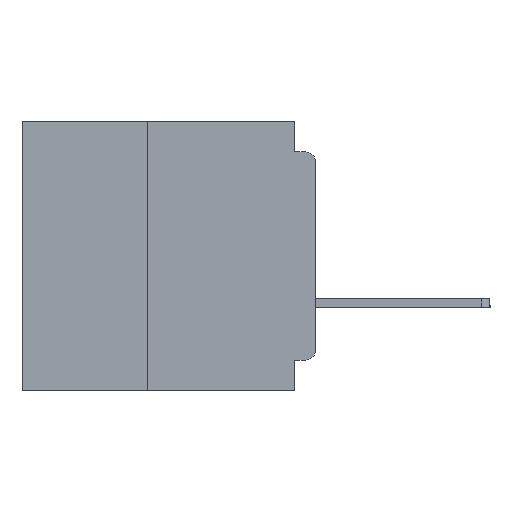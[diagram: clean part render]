
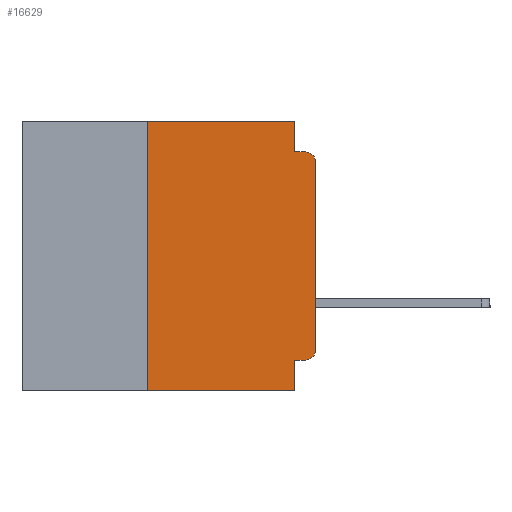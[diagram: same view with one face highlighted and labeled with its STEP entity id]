
A CAD part, left-side view. The second image highlights one B-rep face of the part: STEP entity #16629.
In plain terms, the highlighted planar face has unit normal (-1, 0, 0).
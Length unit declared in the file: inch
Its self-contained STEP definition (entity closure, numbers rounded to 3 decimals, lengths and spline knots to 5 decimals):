
#17 = DIRECTION ( 'NONE',  ( 0., -1., 0. ) ) ;
#1079 = VERTEX_POINT ( 'NONE', #19339 ) ;
#1158 = DIRECTION ( 'NONE',  ( -1., 0., 0. ) ) ;
#1336 = CARTESIAN_POINT ( 'NONE',  ( 0., 0.031, -0.355 ) ) ;
#1384 = CARTESIAN_POINT ( 'NONE',  ( 0., 0., 0. ) ) ;
#1571 = ORIENTED_EDGE ( 'NONE', *, *, #11969, .F. ) ;
#1808 = DIRECTION ( 'NONE',  ( 0., 1., 0. ) ) ;
#1852 = AXIS2_PLACEMENT_3D ( 'NONE', #27922, #35611, #12736 ) ;
#2778 = VECTOR ( 'NONE', #38760, 39.37008 ) ;
#2885 = ORIENTED_EDGE ( 'NONE', *, *, #23136, .F. ) ;
#3098 = LINE ( 'NONE', #1384, #23432 ) ;
#4447 = CARTESIAN_POINT ( 'NONE',  ( 0., 0.015, -0.34 ) ) ;
#4839 = VECTOR ( 'NONE', #40437, 39.37008 ) ;
#5821 = VERTEX_POINT ( 'NONE', #8168 ) ;
#5933 = ORIENTED_EDGE ( 'NONE', *, *, #33757, .F. ) ;
#8168 = CARTESIAN_POINT ( 'NONE',  ( 0., 0., -0.34 ) ) ;
#8252 = DIRECTION ( 'NONE',  ( 0., 0., -1. ) ) ;
#8766 = LINE ( 'NONE', #32472, #38109 ) ;
#8871 = PLANE ( 'NONE',  #1852 ) ;
#10106 = CIRCLE ( 'NONE', #26296, 0.015 ) ;
#10320 = AXIS2_PLACEMENT_3D ( 'NONE', #4447, #31161, #8252 ) ;
#11002 = VERTEX_POINT ( 'NONE', #44364 ) ;
#11969 = EDGE_CURVE ( 'NONE', #32187, #37937, #23117, .T. ) ;
#12736 = DIRECTION ( 'NONE',  ( 0., 0., -1. ) ) ;
#15043 = DIRECTION ( 'NONE',  ( 0., -1., 0. ) ) ;
#15432 = CARTESIAN_POINT ( 'NONE',  ( 0., 0.015, -0.355 ) ) ;
#16629 = ADVANCED_FACE ( 'NONE', ( #44409 ), #8871, .F. ) ;
#16760 = VECTOR ( 'NONE', #15043, 39.37008 ) ;
#17459 = EDGE_CURVE ( 'NONE', #47576, #36792, #35320, .T. ) ;
#19141 = CARTESIAN_POINT ( 'NONE',  ( 0., 0.437, 0. ) ) ;
#19339 = CARTESIAN_POINT ( 'NONE',  ( 0., 0.015, -0.045 ) ) ;
#21579 = VECTOR ( 'NONE', #17, 39.37008 ) ;
#21876 = VECTOR ( 'NONE', #1808, 39.37008 ) ;
#22621 = ORIENTED_EDGE ( 'NONE', *, *, #41962, .F. ) ;
#23117 = LINE ( 'NONE', #34877, #2778 ) ;
#23136 = EDGE_CURVE ( 'NONE', #32006, #32187, #32048, .T. ) ;
#23298 = EDGE_LOOP ( 'NONE', ( #25423, #44460, #47798, #25358, #5933, #22621, #30046, #1571, #2885, #37675 ) ) ;
#23432 = VECTOR ( 'NONE', #47369, 39.37008 ) ;
#24078 = CARTESIAN_POINT ( 'NONE',  ( 0., 0.25, -0.4 ) ) ;
#24091 = CARTESIAN_POINT ( 'NONE',  ( 0., 0.015, -0.06 ) ) ;
#24517 = VERTEX_POINT ( 'NONE', #25801 ) ;
#24734 = CARTESIAN_POINT ( 'NONE',  ( 0., 0., -0.355 ) ) ;
#25358 = ORIENTED_EDGE ( 'NONE', *, *, #17459, .F. ) ;
#25423 = ORIENTED_EDGE ( 'NONE', *, *, #26173, .T. ) ;
#25801 = CARTESIAN_POINT ( 'NONE',  ( 0., 0.25, 0. ) ) ;
#26173 = EDGE_CURVE ( 'NONE', #5821, #11002, #3098, .T. ) ;
#26296 = AXIS2_PLACEMENT_3D ( 'NONE', #24091, #1158, #27927 ) ;
#26949 = EDGE_CURVE ( 'NONE', #36792, #1079, #37111, .T. ) ;
#27922 = CARTESIAN_POINT ( 'NONE',  ( 0., 0.437, 0. ) ) ;
#27927 = DIRECTION ( 'NONE',  ( 0., 0., -1. ) ) ;
#28946 = CARTESIAN_POINT ( 'NONE',  ( 0., 0.25, -0.4 ) ) ;
#30046 = ORIENTED_EDGE ( 'NONE', *, *, #35906, .T. ) ;
#31161 = DIRECTION ( 'NONE',  ( -1., 0., 0. ) ) ;
#31738 = LINE ( 'NONE', #19141, #21579 ) ;
#32006 = VERTEX_POINT ( 'NONE', #15432 ) ;
#32023 = VECTOR ( 'NONE', #46990, 39.37008 ) ;
#32048 = LINE ( 'NONE', #24734, #21876 ) ;
#32187 = VERTEX_POINT ( 'NONE', #1336 ) ;
#32472 = CARTESIAN_POINT ( 'NONE',  ( 0., 0.437, -0.4 ) ) ;
#33757 = EDGE_CURVE ( 'NONE', #24517, #47576, #31738, .T. ) ;
#33858 = EDGE_CURVE ( 'NONE', #32006, #5821, #46095, .T. ) ;
#34877 = CARTESIAN_POINT ( 'NONE',  ( 0., 0.031, -0.4 ) ) ;
#35320 = LINE ( 'NONE', #36733, #4839 ) ;
#35611 = DIRECTION ( 'NONE',  ( 1., 0., 0. ) ) ;
#35906 = EDGE_CURVE ( 'NONE', #37802, #37937, #8766, .T. ) ;
#35992 = CARTESIAN_POINT ( 'NONE',  ( 0., 0.031, 0. ) ) ;
#36307 = DIRECTION ( 'NONE',  ( 0., -1., 0. ) ) ;
#36733 = CARTESIAN_POINT ( 'NONE',  ( 0., 0.031, 0. ) ) ;
#36792 = VERTEX_POINT ( 'NONE', #42609 ) ;
#37111 = LINE ( 'NONE', #37962, #16760 ) ;
#37488 = CARTESIAN_POINT ( 'NONE',  ( 0., 0.031, -0.4 ) ) ;
#37675 = ORIENTED_EDGE ( 'NONE', *, *, #33858, .T. ) ;
#37802 = VERTEX_POINT ( 'NONE', #28946 ) ;
#37937 = VERTEX_POINT ( 'NONE', #37488 ) ;
#37962 = CARTESIAN_POINT ( 'NONE',  ( 0., 0., -0.045 ) ) ;
#38109 = VECTOR ( 'NONE', #36307, 39.37008 ) ;
#38760 = DIRECTION ( 'NONE',  ( 0., 0., -1. ) ) ;
#40437 = DIRECTION ( 'NONE',  ( 0., 0., -1. ) ) ;
#41023 = LINE ( 'NONE', #24078, #32023 ) ;
#41962 = EDGE_CURVE ( 'NONE', #37802, #24517, #41023, .T. ) ;
#42609 = CARTESIAN_POINT ( 'NONE',  ( 0., 0.031, -0.045 ) ) ;
#44364 = CARTESIAN_POINT ( 'NONE',  ( 0., 0., -0.06 ) ) ;
#44409 = FACE_OUTER_BOUND ( 'NONE', #23298, .T. ) ;
#44460 = ORIENTED_EDGE ( 'NONE', *, *, #48062, .T. ) ;
#46095 = CIRCLE ( 'NONE', #10320, 0.015 ) ;
#46990 = DIRECTION ( 'NONE',  ( 0., 0., 1. ) ) ;
#47369 = DIRECTION ( 'NONE',  ( 0., 0., 1. ) ) ;
#47576 = VERTEX_POINT ( 'NONE', #35992 ) ;
#47798 = ORIENTED_EDGE ( 'NONE', *, *, #26949, .F. ) ;
#48062 = EDGE_CURVE ( 'NONE', #11002, #1079, #10106, .T. ) ;
